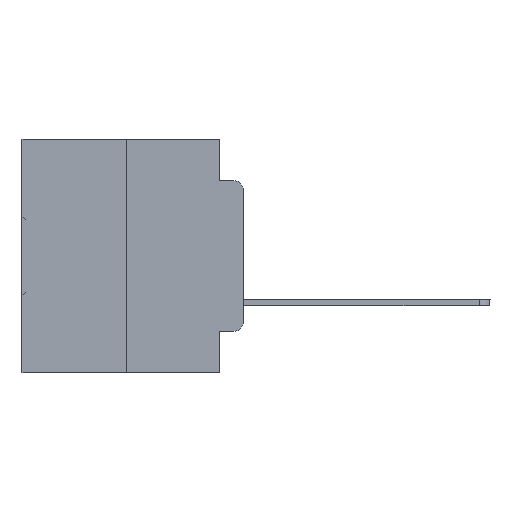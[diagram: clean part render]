
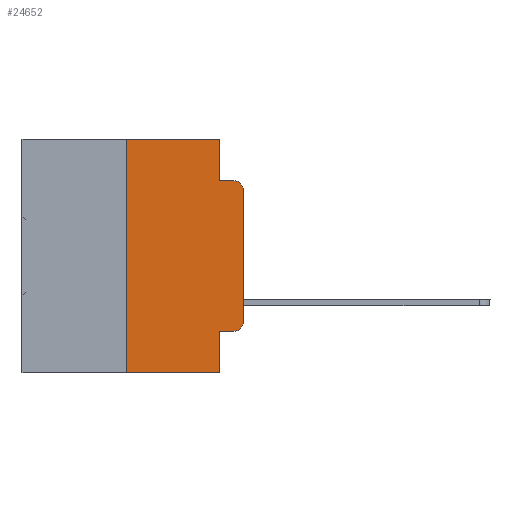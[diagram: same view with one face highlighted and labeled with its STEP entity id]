
A CAD part, left-side view. The second image highlights one B-rep face of the part: STEP entity #24652.
In plain terms, the highlighted planar face has unit normal (-1, 0, 0).
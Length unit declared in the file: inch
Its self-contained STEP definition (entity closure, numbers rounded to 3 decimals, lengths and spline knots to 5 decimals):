
#1518 = VERTEX_POINT ( 'NONE', #16369 ) ;
#1714 = CIRCLE ( 'NONE', #26036, 0.02 ) ;
#2099 = VECTOR ( 'NONE', #23614, 39.37008 ) ;
#2286 = CARTESIAN_POINT ( 'NONE',  ( 0., 0.25, 0. ) ) ;
#2364 = CARTESIAN_POINT ( 'NONE',  ( 0., 0.473, 0. ) ) ;
#3762 = VECTOR ( 'NONE', #14600, 39.37008 ) ;
#4019 = CARTESIAN_POINT ( 'NONE',  ( 0., 0.02, -0.3915 ) ) ;
#4349 = CARTESIAN_POINT ( 'NONE',  ( 0., 0.02, -0.0885 ) ) ;
#4683 = CARTESIAN_POINT ( 'NONE',  ( 0., 0.473, 0. ) ) ;
#4852 = LINE ( 'NONE', #4683, #2099 ) ;
#4894 = AXIS2_PLACEMENT_3D ( 'NONE', #19018, #5926, #22031 ) ;
#5076 = VERTEX_POINT ( 'NONE', #4349 ) ;
#5211 = LINE ( 'NONE', #25366, #34150 ) ;
#5926 = DIRECTION ( 'NONE',  ( -1., 0., 0. ) ) ;
#6337 = ORIENTED_EDGE ( 'NONE', *, *, #28044, .F. ) ;
#6560 = VERTEX_POINT ( 'NONE', #22722 ) ;
#6679 = LINE ( 'NONE', #20850, #14738 ) ;
#7030 = CARTESIAN_POINT ( 'NONE',  ( 0., 0.051, 0. ) ) ;
#7667 = FACE_OUTER_BOUND ( 'NONE', #14002, .T. ) ;
#8142 = CARTESIAN_POINT ( 'NONE',  ( 0., 0.051, -0.0885 ) ) ;
#8165 = ORIENTED_EDGE ( 'NONE', *, *, #9826, .F. ) ;
#8272 = ORIENTED_EDGE ( 'NONE', *, *, #25751, .T. ) ;
#9687 = LINE ( 'NONE', #7030, #25086 ) ;
#9826 = EDGE_CURVE ( 'NONE', #11500, #5076, #32206, .T. ) ;
#11500 = VERTEX_POINT ( 'NONE', #30407 ) ;
#12526 = DIRECTION ( 'NONE',  ( 0., 0., -1. ) ) ;
#12627 = ORIENTED_EDGE ( 'NONE', *, *, #26278, .T. ) ;
#12852 = VERTEX_POINT ( 'NONE', #30758 ) ;
#12941 = EDGE_CURVE ( 'NONE', #17153, #11500, #6679, .T. ) ;
#13126 = LINE ( 'NONE', #23926, #17348 ) ;
#13163 = DIRECTION ( 'NONE',  ( 0., 0., -1. ) ) ;
#13813 = CARTESIAN_POINT ( 'NONE',  ( 0., 0.051, 0. ) ) ;
#14002 = EDGE_LOOP ( 'NONE', ( #12627, #25329, #8165, #14799, #32360, #6337, #17028, #27369, #8272, #18196 ) ) ;
#14564 = CARTESIAN_POINT ( 'NONE',  ( 0., 0., -0.3915 ) ) ;
#14600 = DIRECTION ( 'NONE',  ( 0., -1., 0. ) ) ;
#14738 = VECTOR ( 'NONE', #28826, 39.37008 ) ;
#14799 = ORIENTED_EDGE ( 'NONE', *, *, #12941, .F. ) ;
#16329 = VECTOR ( 'NONE', #18928, 39.37008 ) ;
#16369 = CARTESIAN_POINT ( 'NONE',  ( 0., 0.051, -0.4115 ) ) ;
#16525 = EDGE_CURVE ( 'NONE', #17170, #34713, #1714, .T. ) ;
#17028 = ORIENTED_EDGE ( 'NONE', *, *, #22157, .T. ) ;
#17153 = VERTEX_POINT ( 'NONE', #13813 ) ;
#17170 = VERTEX_POINT ( 'NONE', #26296 ) ;
#17348 = VECTOR ( 'NONE', #32216, 39.37008 ) ;
#18196 = ORIENTED_EDGE ( 'NONE', *, *, #16525, .T. ) ;
#18515 = DIRECTION ( 'NONE',  ( 0., 0., -1. ) ) ;
#18928 = DIRECTION ( 'NONE',  ( 0., -1., 0. ) ) ;
#19018 = CARTESIAN_POINT ( 'NONE',  ( 0., 0.02, -0.1085 ) ) ;
#20084 = AXIS2_PLACEMENT_3D ( 'NONE', #2364, #28935, #13163 ) ;
#20850 = CARTESIAN_POINT ( 'NONE',  ( 0., 0.051, 0. ) ) ;
#21225 = LINE ( 'NONE', #2286, #32646 ) ;
#21493 = EDGE_CURVE ( 'NONE', #1518, #6560, #9687, .T. ) ;
#22031 = DIRECTION ( 'NONE',  ( 0., 0., -1. ) ) ;
#22157 = EDGE_CURVE ( 'NONE', #12852, #6560, #5211, .T. ) ;
#22187 = DIRECTION ( 'NONE',  ( 0., -1., 0. ) ) ;
#22722 = CARTESIAN_POINT ( 'NONE',  ( 0., 0.051, -0.5 ) ) ;
#23496 = DIRECTION ( 'NONE',  ( -1., 0., 0. ) ) ;
#23614 = DIRECTION ( 'NONE',  ( 0., -1., 0. ) ) ;
#23926 = CARTESIAN_POINT ( 'NONE',  ( 0., 0., 0. ) ) ;
#24592 = EDGE_CURVE ( 'NONE', #34019, #17153, #4852, .T. ) ;
#24652 = ADVANCED_FACE ( 'NONE', ( #7667 ), #26800, .F. ) ;
#25086 = VECTOR ( 'NONE', #18515, 39.37008 ) ;
#25329 = ORIENTED_EDGE ( 'NONE', *, *, #25569, .T. ) ;
#25366 = CARTESIAN_POINT ( 'NONE',  ( 0., 0.473, -0.5 ) ) ;
#25398 = CARTESIAN_POINT ( 'NONE',  ( 0., 0.051, -0.4115 ) ) ;
#25487 = CARTESIAN_POINT ( 'NONE',  ( 0., 0., -0.1085 ) ) ;
#25569 = EDGE_CURVE ( 'NONE', #27955, #5076, #33675, .T. ) ;
#25751 = EDGE_CURVE ( 'NONE', #1518, #17170, #28056, .T. ) ;
#26036 = AXIS2_PLACEMENT_3D ( 'NONE', #4019, #23496, #12526 ) ;
#26278 = EDGE_CURVE ( 'NONE', #34713, #27955, #13126, .T. ) ;
#26296 = CARTESIAN_POINT ( 'NONE',  ( 0., 0.02, -0.4115 ) ) ;
#26800 = PLANE ( 'NONE',  #20084 ) ;
#27369 = ORIENTED_EDGE ( 'NONE', *, *, #21493, .F. ) ;
#27955 = VERTEX_POINT ( 'NONE', #25487 ) ;
#28044 = EDGE_CURVE ( 'NONE', #12852, #34019, #21225, .T. ) ;
#28056 = LINE ( 'NONE', #25398, #3762 ) ;
#28826 = DIRECTION ( 'NONE',  ( 0., 0., -1. ) ) ;
#28935 = DIRECTION ( 'NONE',  ( 1., 0., 0. ) ) ;
#30407 = CARTESIAN_POINT ( 'NONE',  ( 0., 0.051, -0.0885 ) ) ;
#30758 = CARTESIAN_POINT ( 'NONE',  ( 0., 0.25, -0.5 ) ) ;
#31313 = DIRECTION ( 'NONE',  ( 0., 0., 1. ) ) ;
#32206 = LINE ( 'NONE', #8142, #16329 ) ;
#32216 = DIRECTION ( 'NONE',  ( 0., 0., 1. ) ) ;
#32360 = ORIENTED_EDGE ( 'NONE', *, *, #24592, .F. ) ;
#32646 = VECTOR ( 'NONE', #31313, 39.37008 ) ;
#33675 = CIRCLE ( 'NONE', #4894, 0.02 ) ;
#34019 = VERTEX_POINT ( 'NONE', #34126 ) ;
#34126 = CARTESIAN_POINT ( 'NONE',  ( 0., 0.25, 0. ) ) ;
#34150 = VECTOR ( 'NONE', #22187, 39.37008 ) ;
#34713 = VERTEX_POINT ( 'NONE', #14564 ) ;
